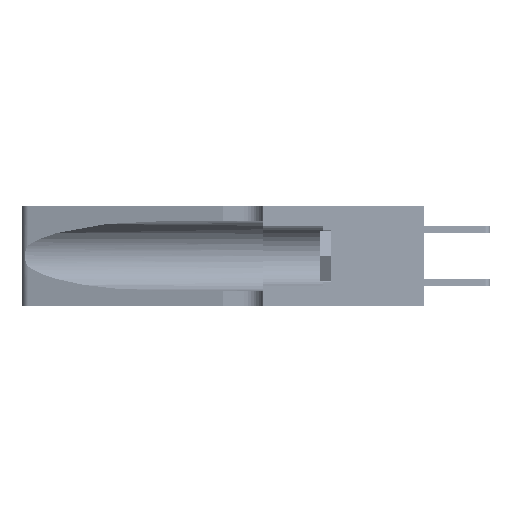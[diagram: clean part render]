
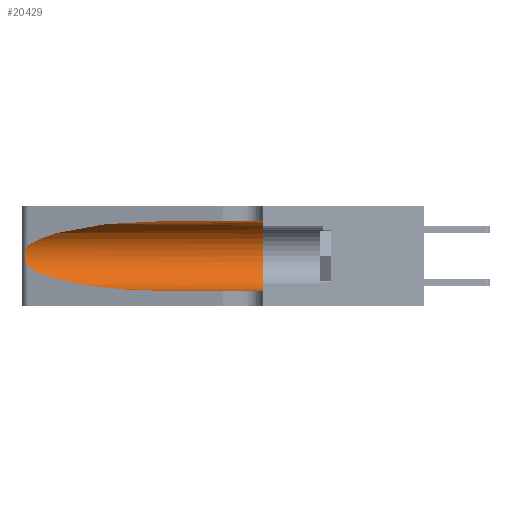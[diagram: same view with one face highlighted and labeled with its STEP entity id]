
A CAD part, left-side view. The second image highlights one B-rep face of the part: STEP entity #20429.
In plain terms, the highlighted cylindrical face has radius 3.308 mm (diameter 6.617 mm), a partial arc.
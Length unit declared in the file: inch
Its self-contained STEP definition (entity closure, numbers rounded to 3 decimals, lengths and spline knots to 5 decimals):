
#90 = ORIENTED_EDGE ( 'NONE', *, *, #7128, .F. ) ;
#395 = VERTEX_POINT ( 'NONE', #34033 ) ;
#1290 = CARTESIAN_POINT ( 'NONE',  ( 0.25854, 1.2359, 0.20912 ) ) ;
#1416 = CARTESIAN_POINT ( 'NONE',  ( 0.26075, 1.23896, 0.178 ) ) ;
#1712 = CARTESIAN_POINT ( 'NONE',  ( 0.26075, 1.23896, 0.19203 ) ) ;
#2355 = ORIENTED_EDGE ( 'NONE', *, *, #28344, .T. ) ;
#3023 = DIRECTION ( 'NONE',  ( 0., 0., 1. ) ) ;
#3497 = CARTESIAN_POINT ( 'NONE',  ( 0.25487, 1.22718, 0.14631 ) ) ;
#4100 = EDGE_CURVE ( 'NONE', #5969, #18372, #14498, .T. ) ;
#5061 = CARTESIAN_POINT ( 'NONE',  ( 0.25487, 1.22718, 0.22369 ) ) ;
#5086 = CARTESIAN_POINT ( 'NONE',  ( 0.25856, 1.23593, 0.16098 ) ) ;
#5389 = FACE_OUTER_BOUND ( 'NONE', #36159, .T. ) ;
#5535 = VECTOR ( 'NONE', #35222, 39.37008 ) ;
#5782 = CARTESIAN_POINT ( 'NONE',  ( 0.25487, 1.22718, 0.14631 ) ) ;
#5969 = VERTEX_POINT ( 'NONE', #37720 ) ;
#5990 = CARTESIAN_POINT ( 'NONE',  ( 0.1305, 0.35, 0.185 ) ) ;
#6169 = ORIENTED_EDGE ( 'NONE', *, *, #31128, .T. ) ;
#6214 = CARTESIAN_POINT ( 'NONE',  ( 0.25555, 1.22993, 0.14849 ) ) ;
#6423 = ORIENTED_EDGE ( 'NONE', *, *, #22171, .F. ) ;
#6571 = DIRECTION ( 'NONE',  ( 0., 1., 0. ) ) ;
#7128 = EDGE_CURVE ( 'NONE', #41959, #395, #36518, .T. ) ;
#7487 = CYLINDRICAL_SURFACE ( 'NONE', #20344, 0.13025 ) ;
#7602 = ORIENTED_EDGE ( 'NONE', *, *, #8664, .T. ) ;
#7729 = DIRECTION ( 'NONE',  ( 0., -1., 0. ) ) ;
#8321 = CARTESIAN_POINT ( 'NONE',  ( 0.25555, 1.22994, 0.2215 ) ) ;
#8664 = EDGE_CURVE ( 'NONE', #41959, #5969, #13139, .T. ) ;
#9191 = CARTESIAN_POINT ( 'NONE',  ( 0.1305, 0.72297, 0.05475 ) ) ;
#10745 = CARTESIAN_POINT ( 'NONE',  ( 0.1305, 0.35, 0.05475 ) ) ;
#11030 = VERTEX_POINT ( 'NONE', #10745 ) ;
#11696 = CARTESIAN_POINT ( 'NONE',  ( 0.2373, 1.15595, 0.28018 ) ) ;
#12329 = LINE ( 'NONE', #24380, #40144 ) ;
#13139 =( BOUNDED_CURVE ( )  B_SPLINE_CURVE ( 3, ( #38106, #31651, #11696, #5061 ),
 .UNSPECIFIED., .F., .T. ) 
 B_SPLINE_CURVE_WITH_KNOTS ( ( 4, 4 ),
 ( 1.5708, 2.84003 ),
 .UNSPECIFIED. ) 
 CURVE ( )  GEOMETRIC_REPRESENTATION_ITEM ( )  RATIONAL_B_SPLINE_CURVE ( ( 1., 0.87, 0.87, 1. ) ) 
 REPRESENTATION_ITEM ( '' )  );
#14498 = B_SPLINE_CURVE_WITH_KNOTS ( 'NONE', 3,
 ( #28470, #8321, #35207, #14553, #1290, #41644, #1712, #1416, #25256, #5086, #34629, #37997, #6214, #5782 ),
 .UNSPECIFIED., .F., .F.,
 ( 4, 2, 2, 2, 2, 2, 4 ),
 ( 0., 0.00027, 0.00053, 0.00107, 0.0016, 0.00187, 0.00214 ),
 .UNSPECIFIED. ) ;
#14553 = CARTESIAN_POINT ( 'NONE',  ( 0.25787, 1.23484, 0.2124 ) ) ;
#18273 = ORIENTED_EDGE ( 'NONE', *, *, #4100, .T. ) ;
#18372 = VERTEX_POINT ( 'NONE', #3497 ) ;
#20344 = AXIS2_PLACEMENT_3D ( 'NONE', #24225, #27551, #41174 ) ;
#20429 = ADVANCED_FACE ( 'NONE', ( #5389 ), #7487, .F. ) ;
#22171 = EDGE_CURVE ( 'NONE', #395, #11030, #27287, .T. ) ;
#24225 = CARTESIAN_POINT ( 'NONE',  ( 0.1305, 1.61858, 0.185 ) ) ;
#24380 = CARTESIAN_POINT ( 'NONE',  ( 0.1305, 1.61858, 0.05475 ) ) ;
#25256 = CARTESIAN_POINT ( 'NONE',  ( 0.26017, 1.23833, 0.17102 ) ) ;
#26843 =( BOUNDED_CURVE ( )  B_SPLINE_CURVE ( 3, ( #29468, #32832, #36210, #9191 ),
 .UNSPECIFIED., .F., .F. ) 
 B_SPLINE_CURVE_WITH_KNOTS ( ( 4, 4 ),
 ( 3.44316, 4.71239 ),
 .UNSPECIFIED. ) 
 CURVE ( )  GEOMETRIC_REPRESENTATION_ITEM ( )  RATIONAL_B_SPLINE_CURVE ( ( 1., 0.87, 0.87, 1. ) ) 
 REPRESENTATION_ITEM ( '' )  );
#27287 = CIRCLE ( 'NONE', #42245, 0.13025 ) ;
#27440 = CARTESIAN_POINT ( 'NONE',  ( 0.1305, 0.72297, 0.31525 ) ) ;
#27551 = DIRECTION ( 'NONE',  ( 0., -1., 0. ) ) ;
#28344 = EDGE_CURVE ( 'NONE', #36456, #11030, #12329, .T. ) ;
#28470 = CARTESIAN_POINT ( 'NONE',  ( 0.25487, 1.22718, 0.22369 ) ) ;
#28489 = CARTESIAN_POINT ( 'NONE',  ( 0.1305, 1.61858, 0.31525 ) ) ;
#29468 = CARTESIAN_POINT ( 'NONE',  ( 0.25487, 1.22718, 0.14631 ) ) ;
#30422 = CARTESIAN_POINT ( 'NONE',  ( 0.1305, 0.72297, 0.05475 ) ) ;
#31128 = EDGE_CURVE ( 'NONE', #18372, #36456, #26843, .T. ) ;
#31651 = CARTESIAN_POINT ( 'NONE',  ( 0.18966, 0.96281, 0.31525 ) ) ;
#32832 = CARTESIAN_POINT ( 'NONE',  ( 0.2373, 1.15595, 0.08982 ) ) ;
#34033 = CARTESIAN_POINT ( 'NONE',  ( 0.1305, 0.35, 0.31525 ) ) ;
#34629 = CARTESIAN_POINT ( 'NONE',  ( 0.25789, 1.23486, 0.15765 ) ) ;
#35207 = CARTESIAN_POINT ( 'NONE',  ( 0.25639, 1.23184, 0.21858 ) ) ;
#35222 = DIRECTION ( 'NONE',  ( 0., -1., 0. ) ) ;
#36159 = EDGE_LOOP ( 'NONE', ( #7602, #18273, #6169, #2355, #6423, #90 ) ) ;
#36210 = CARTESIAN_POINT ( 'NONE',  ( 0.18966, 0.96281, 0.05475 ) ) ;
#36456 = VERTEX_POINT ( 'NONE', #30422 ) ;
#36518 = LINE ( 'NONE', #28489, #5535 ) ;
#37720 = CARTESIAN_POINT ( 'NONE',  ( 0.25487, 1.22718, 0.22369 ) ) ;
#37997 = CARTESIAN_POINT ( 'NONE',  ( 0.25639, 1.23186, 0.15144 ) ) ;
#38106 = CARTESIAN_POINT ( 'NONE',  ( 0.1305, 0.72297, 0.31525 ) ) ;
#40144 = VECTOR ( 'NONE', #7729, 39.37008 ) ;
#41174 = DIRECTION ( 'NONE',  ( 0., 0., -1. ) ) ;
#41644 = CARTESIAN_POINT ( 'NONE',  ( 0.26018, 1.23835, 0.19895 ) ) ;
#41959 = VERTEX_POINT ( 'NONE', #27440 ) ;
#42245 = AXIS2_PLACEMENT_3D ( 'NONE', #5990, #6571, #3023 ) ;
